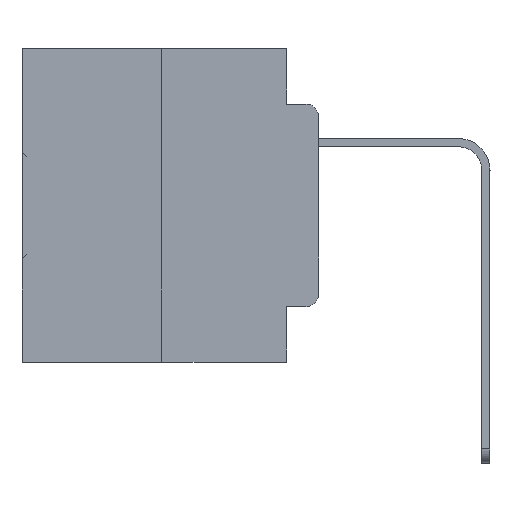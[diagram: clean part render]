
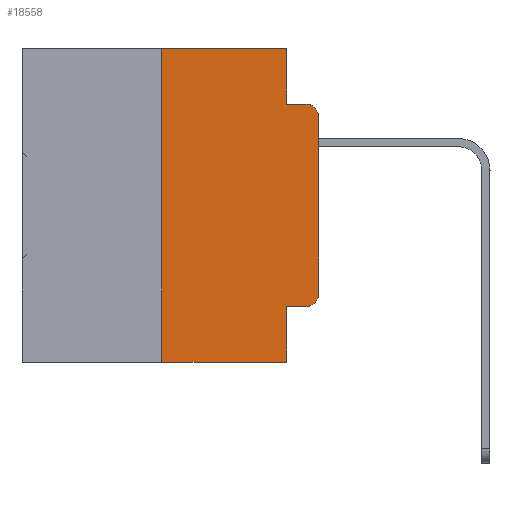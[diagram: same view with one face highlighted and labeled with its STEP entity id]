
A CAD part, left-side view. The second image highlights one B-rep face of the part: STEP entity #18558.
In plain terms, the highlighted planar face has unit normal (-1, 0, 0).
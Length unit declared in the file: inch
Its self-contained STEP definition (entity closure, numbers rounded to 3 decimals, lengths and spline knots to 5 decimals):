
#880 = ORIENTED_EDGE ( 'NONE', *, *, #15516, .F. ) ;
#1437 = VECTOR ( 'NONE', #30553, 39.37008 ) ;
#1526 = CARTESIAN_POINT ( 'NONE',  ( 0., 0., 0. ) ) ;
#1776 = EDGE_LOOP ( 'NONE', ( #8193, #5344, #880, #10071, #16179, #34741, #25386, #18137, #22469, #18712 ) ) ;
#2642 = CARTESIAN_POINT ( 'NONE',  ( 0., 0.25, -0.5 ) ) ;
#2724 = CARTESIAN_POINT ( 'NONE',  ( 0., 0.051, -0.4115 ) ) ;
#2725 = LINE ( 'NONE', #24805, #15901 ) ;
#3711 = CARTESIAN_POINT ( 'NONE',  ( 0., 0.051, -0.4115 ) ) ;
#4463 = EDGE_CURVE ( 'NONE', #34296, #15541, #20231, .T. ) ;
#4544 = DIRECTION ( 'NONE',  ( 0., 0., -1. ) ) ;
#5344 = ORIENTED_EDGE ( 'NONE', *, *, #21570, .T. ) ;
#5555 = CARTESIAN_POINT ( 'NONE',  ( 0., 0.051, -0.5 ) ) ;
#5573 = CIRCLE ( 'NONE', #17705, 0.02 ) ;
#5845 = CARTESIAN_POINT ( 'NONE',  ( 0., 0.473, 0. ) ) ;
#6168 = VECTOR ( 'NONE', #28844, 39.37008 ) ;
#6252 = EDGE_CURVE ( 'NONE', #30354, #30837, #27247, .T. ) ;
#7184 = CARTESIAN_POINT ( 'NONE',  ( 0., 0.25, 0. ) ) ;
#7703 = VECTOR ( 'NONE', #22856, 39.37008 ) ;
#8193 = ORIENTED_EDGE ( 'NONE', *, *, #11010, .T. ) ;
#9561 = CARTESIAN_POINT ( 'NONE',  ( 0., 0., -0.1085 ) ) ;
#10071 = ORIENTED_EDGE ( 'NONE', *, *, #18165, .F. ) ;
#10471 = LINE ( 'NONE', #16590, #13430 ) ;
#11010 = EDGE_CURVE ( 'NONE', #14187, #25714, #30989, .T. ) ;
#11516 = VECTOR ( 'NONE', #31082, 39.37008 ) ;
#11943 = LINE ( 'NONE', #23193, #7703 ) ;
#12800 = VERTEX_POINT ( 'NONE', #16569 ) ;
#13150 = DIRECTION ( 'NONE',  ( -1., 0., 0. ) ) ;
#13430 = VECTOR ( 'NONE', #27489, 39.37008 ) ;
#13646 = VECTOR ( 'NONE', #22438, 39.37008 ) ;
#13948 = VERTEX_POINT ( 'NONE', #29846 ) ;
#14187 = VERTEX_POINT ( 'NONE', #28304 ) ;
#14274 = DIRECTION ( 'NONE',  ( 0., 0., -1. ) ) ;
#15516 = EDGE_CURVE ( 'NONE', #13948, #18988, #32005, .T. ) ;
#15541 = VERTEX_POINT ( 'NONE', #7184 ) ;
#15901 = VECTOR ( 'NONE', #14274, 39.37008 ) ;
#16179 = ORIENTED_EDGE ( 'NONE', *, *, #34080, .F. ) ;
#16569 = CARTESIAN_POINT ( 'NONE',  ( 0., 0.051, 0. ) ) ;
#16590 = CARTESIAN_POINT ( 'NONE',  ( 0., 0.473, -0.5 ) ) ;
#17705 = AXIS2_PLACEMENT_3D ( 'NONE', #29237, #13150, #21247 ) ;
#17852 = VERTEX_POINT ( 'NONE', #5555 ) ;
#17878 = FACE_OUTER_BOUND ( 'NONE', #1776, .T. ) ;
#18137 = ORIENTED_EDGE ( 'NONE', *, *, #33007, .F. ) ;
#18165 = EDGE_CURVE ( 'NONE', #12800, #13948, #11943, .T. ) ;
#18176 = AXIS2_PLACEMENT_3D ( 'NONE', #32386, #35003, #29315 ) ;
#18558 = ADVANCED_FACE ( 'NONE', ( #17878 ), #32260, .F. ) ;
#18712 = ORIENTED_EDGE ( 'NONE', *, *, #26621, .T. ) ;
#18827 = LINE ( 'NONE', #5845, #1437 ) ;
#18988 = VERTEX_POINT ( 'NONE', #23506 ) ;
#20231 = LINE ( 'NONE', #33054, #13646 ) ;
#21247 = DIRECTION ( 'NONE',  ( 0., 0., -1. ) ) ;
#21570 = EDGE_CURVE ( 'NONE', #25714, #18988, #34403, .T. ) ;
#22438 = DIRECTION ( 'NONE',  ( 0., 0., 1. ) ) ;
#22469 = ORIENTED_EDGE ( 'NONE', *, *, #6252, .T. ) ;
#22856 = DIRECTION ( 'NONE',  ( 0., 0., -1. ) ) ;
#23162 = CARTESIAN_POINT ( 'NONE',  ( 0., 0.02, -0.1085 ) ) ;
#23193 = CARTESIAN_POINT ( 'NONE',  ( 0., 0.051, 0. ) ) ;
#23272 = DIRECTION ( 'NONE',  ( -1., 0., 0. ) ) ;
#23431 = VECTOR ( 'NONE', #27990, 39.37008 ) ;
#23506 = CARTESIAN_POINT ( 'NONE',  ( 0., 0.02, -0.0885 ) ) ;
#24805 = CARTESIAN_POINT ( 'NONE',  ( 0., 0.051, 0. ) ) ;
#25386 = ORIENTED_EDGE ( 'NONE', *, *, #31712, .T. ) ;
#25714 = VERTEX_POINT ( 'NONE', #9561 ) ;
#26621 = EDGE_CURVE ( 'NONE', #30837, #14187, #5573, .T. ) ;
#27221 = CARTESIAN_POINT ( 'NONE',  ( 0., 0.02, -0.4115 ) ) ;
#27247 = LINE ( 'NONE', #3711, #23431 ) ;
#27489 = DIRECTION ( 'NONE',  ( 0., -1., 0. ) ) ;
#27990 = DIRECTION ( 'NONE',  ( 0., -1., 0. ) ) ;
#28304 = CARTESIAN_POINT ( 'NONE',  ( 0., 0., -0.3915 ) ) ;
#28844 = DIRECTION ( 'NONE',  ( 0., -1., 0. ) ) ;
#29237 = CARTESIAN_POINT ( 'NONE',  ( 0., 0.02, -0.3915 ) ) ;
#29315 = DIRECTION ( 'NONE',  ( 0., 0., -1. ) ) ;
#29846 = CARTESIAN_POINT ( 'NONE',  ( 0., 0.051, -0.0885 ) ) ;
#30205 = AXIS2_PLACEMENT_3D ( 'NONE', #23162, #23272, #4544 ) ;
#30354 = VERTEX_POINT ( 'NONE', #2724 ) ;
#30553 = DIRECTION ( 'NONE',  ( 0., -1., 0. ) ) ;
#30837 = VERTEX_POINT ( 'NONE', #27221 ) ;
#30989 = LINE ( 'NONE', #1526, #11516 ) ;
#31082 = DIRECTION ( 'NONE',  ( 0., 0., 1. ) ) ;
#31429 = CARTESIAN_POINT ( 'NONE',  ( 0., 0.051, -0.0885 ) ) ;
#31712 = EDGE_CURVE ( 'NONE', #34296, #17852, #10471, .T. ) ;
#32005 = LINE ( 'NONE', #31429, #6168 ) ;
#32260 = PLANE ( 'NONE',  #18176 ) ;
#32386 = CARTESIAN_POINT ( 'NONE',  ( 0., 0.473, 0. ) ) ;
#33007 = EDGE_CURVE ( 'NONE', #30354, #17852, #2725, .T. ) ;
#33054 = CARTESIAN_POINT ( 'NONE',  ( 0., 0.25, 0. ) ) ;
#34080 = EDGE_CURVE ( 'NONE', #15541, #12800, #18827, .T. ) ;
#34296 = VERTEX_POINT ( 'NONE', #2642 ) ;
#34403 = CIRCLE ( 'NONE', #30205, 0.02 ) ;
#34741 = ORIENTED_EDGE ( 'NONE', *, *, #4463, .F. ) ;
#35003 = DIRECTION ( 'NONE',  ( 1., 0., 0. ) ) ;
